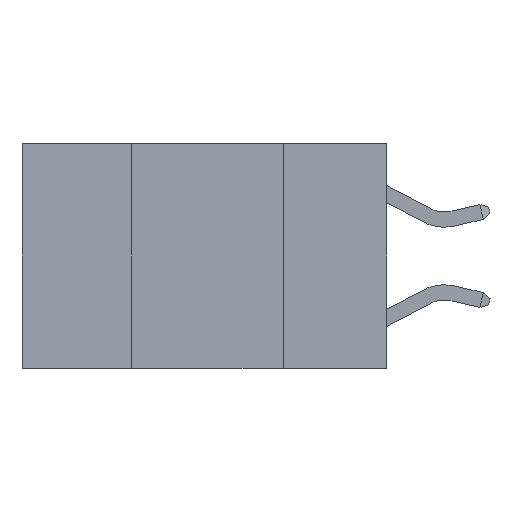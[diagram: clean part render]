
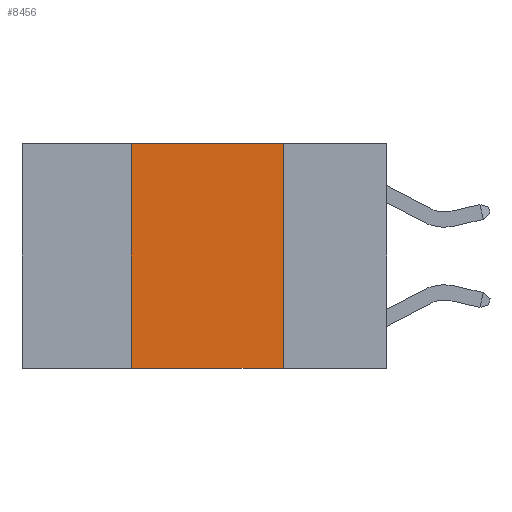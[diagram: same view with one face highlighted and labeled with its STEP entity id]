
A CAD part, left-side view. The second image highlights one B-rep face of the part: STEP entity #8456.
In plain terms, the highlighted planar face has unit normal (-1, 0, 0).
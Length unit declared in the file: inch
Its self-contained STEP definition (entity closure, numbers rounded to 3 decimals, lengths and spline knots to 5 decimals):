
#363 = LINE ( 'NONE', #4498, #2870 ) ;
#674 = CARTESIAN_POINT ( 'NONE',  ( 0., 0.6, 0. ) ) ;
#689 = LINE ( 'NONE', #3281, #10014 ) ;
#1710 = DIRECTION ( 'NONE',  ( 0., -1., 0. ) ) ;
#1746 = CARTESIAN_POINT ( 'NONE',  ( 0., 0.42, 0. ) ) ;
#2346 = DIRECTION ( 'NONE',  ( 0., 0., 1. ) ) ;
#2870 = VECTOR ( 'NONE', #1710, 39.37008 ) ;
#3027 = LINE ( 'NONE', #5515, #9862 ) ;
#3281 = CARTESIAN_POINT ( 'NONE',  ( 0., 0.42, 0. ) ) ;
#3490 = PLANE ( 'NONE',  #11216 ) ;
#4410 = DIRECTION ( 'NONE',  ( 0., 0., -1. ) ) ;
#4452 = ORIENTED_EDGE ( 'NONE', *, *, #9103, .T. ) ;
#4498 = CARTESIAN_POINT ( 'NONE',  ( 0., 0.6, 0. ) ) ;
#5441 = ORIENTED_EDGE ( 'NONE', *, *, #9888, .F. ) ;
#5515 = CARTESIAN_POINT ( 'NONE',  ( 0., 0.6, -0.37 ) ) ;
#5693 = CARTESIAN_POINT ( 'NONE',  ( 0., 0.17, 0. ) ) ;
#6558 = CARTESIAN_POINT ( 'NONE',  ( 0., 0.42, -0.37 ) ) ;
#6571 = DIRECTION ( 'NONE',  ( 0., 0., -1. ) ) ;
#6924 = CARTESIAN_POINT ( 'NONE',  ( 0., 0.17, -0.37 ) ) ;
#7175 = VERTEX_POINT ( 'NONE', #6558 ) ;
#7441 = VERTEX_POINT ( 'NONE', #6924 ) ;
#8456 = ADVANCED_FACE ( 'NONE', ( #9740 ), #3490, .F. ) ;
#8544 = LINE ( 'NONE', #5693, #10429 ) ;
#8879 = EDGE_CURVE ( 'NONE', #7175, #9718, #689, .T. ) ;
#9103 = EDGE_CURVE ( 'NONE', #7175, #7441, #3027, .T. ) ;
#9208 = DIRECTION ( 'NONE',  ( 0., -1., 0. ) ) ;
#9358 = EDGE_LOOP ( 'NONE', ( #5441, #12016, #10839, #4452 ) ) ;
#9689 = EDGE_CURVE ( 'NONE', #9718, #11027, #363, .T. ) ;
#9718 = VERTEX_POINT ( 'NONE', #1746 ) ;
#9740 = FACE_OUTER_BOUND ( 'NONE', #9358, .T. ) ;
#9862 = VECTOR ( 'NONE', #9208, 39.37008 ) ;
#9888 = EDGE_CURVE ( 'NONE', #11027, #7441, #8544, .T. ) ;
#10001 = DIRECTION ( 'NONE',  ( 1., 0., 0. ) ) ;
#10014 = VECTOR ( 'NONE', #2346, 39.37008 ) ;
#10429 = VECTOR ( 'NONE', #6571, 39.37008 ) ;
#10839 = ORIENTED_EDGE ( 'NONE', *, *, #8879, .F. ) ;
#11027 = VERTEX_POINT ( 'NONE', #11693 ) ;
#11216 = AXIS2_PLACEMENT_3D ( 'NONE', #674, #10001, #4410 ) ;
#11693 = CARTESIAN_POINT ( 'NONE',  ( 0., 0.17, 0. ) ) ;
#12016 = ORIENTED_EDGE ( 'NONE', *, *, #9689, .F. ) ;
